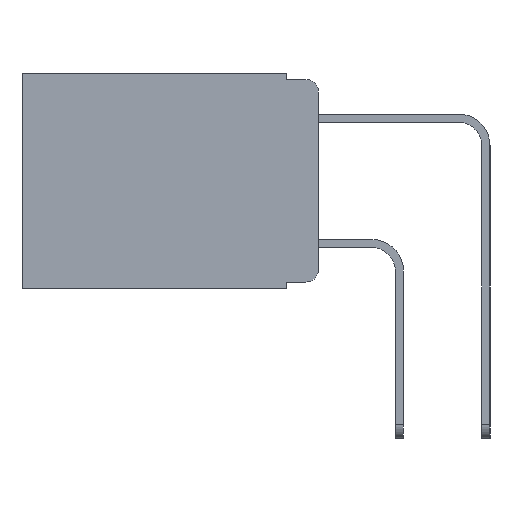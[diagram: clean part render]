
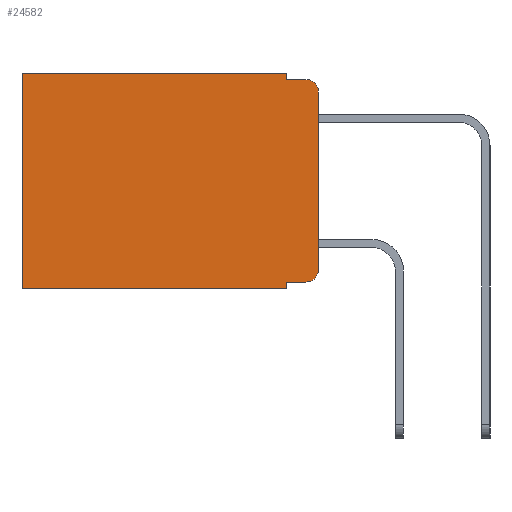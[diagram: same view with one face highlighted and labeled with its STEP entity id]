
A CAD part, left-side view. The second image highlights one B-rep face of the part: STEP entity #24582.
In plain terms, the highlighted planar face has unit normal (-1, 0, 0).
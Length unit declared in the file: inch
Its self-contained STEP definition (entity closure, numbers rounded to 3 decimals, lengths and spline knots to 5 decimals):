
#254 = PLANE ( 'NONE',  #23948 ) ;
#559 = LINE ( 'NONE', #24559, #5121 ) ;
#582 = VECTOR ( 'NONE', #24041, 39.37008 ) ;
#994 = EDGE_CURVE ( 'NONE', #19160, #9519, #16504, .T. ) ;
#1526 = DIRECTION ( 'NONE',  ( 0., 0., -1. ) ) ;
#1638 = EDGE_LOOP ( 'NONE', ( #12929, #13010, #13178, #13196, #13227, #13409, #13428, #13522, #13635, #13654 ) ) ;
#1689 = FACE_OUTER_BOUND ( 'NONE', #1638, .T. ) ;
#1794 = DIRECTION ( 'NONE',  ( -1., 0., 0. ) ) ;
#2107 = VERTEX_POINT ( 'NONE', #8570 ) ;
#2148 = CARTESIAN_POINT ( 'NONE',  ( 0.298, 0.051, 0. ) ) ;
#2186 = AXIS2_PLACEMENT_3D ( 'NONE', #14984, #3344, #16945 ) ;
#2248 = DIRECTION ( 'NONE',  ( 1., 0., 0. ) ) ;
#2664 = VECTOR ( 'NONE', #23885, 39.37008 ) ;
#2675 = CARTESIAN_POINT ( 'NONE',  ( 0.298, 0.051, -0.333 ) ) ;
#2977 = EDGE_CURVE ( 'NONE', #10206, #17393, #21224, .T. ) ;
#2984 = CARTESIAN_POINT ( 'NONE',  ( 0.298, 0.051, -0.343 ) ) ;
#3323 = VECTOR ( 'NONE', #3538, 39.37008 ) ;
#3344 = DIRECTION ( 'NONE',  ( -1., 0., 0. ) ) ;
#3425 = EDGE_CURVE ( 'NONE', #9216, #24380, #559, .T. ) ;
#3452 = CARTESIAN_POINT ( 'NONE',  ( 0.298, 0.473, 0. ) ) ;
#3538 = DIRECTION ( 'NONE',  ( 0., 0., -1. ) ) ;
#3616 = EDGE_CURVE ( 'NONE', #2107, #9216, #21827, .T. ) ;
#4163 = EDGE_CURVE ( 'NONE', #9519, #13200, #4528, .T. ) ;
#4528 = LINE ( 'NONE', #11859, #19377 ) ;
#5121 = VECTOR ( 'NONE', #23825, 39.37008 ) ;
#6774 = VECTOR ( 'NONE', #1526, 39.37008 ) ;
#6919 = VECTOR ( 'NONE', #9480, 39.37008 ) ;
#7004 = VERTEX_POINT ( 'NONE', #14033 ) ;
#7548 = DIRECTION ( 'NONE',  ( 0., 0., -1. ) ) ;
#7786 = EDGE_CURVE ( 'NONE', #10090, #24380, #18799, .T. ) ;
#8004 = CARTESIAN_POINT ( 'NONE',  ( 0.298, 0., 0. ) ) ;
#8570 = CARTESIAN_POINT ( 'NONE',  ( 0.298, 0.051, -0.333 ) ) ;
#8912 = DIRECTION ( 'NONE',  ( 0., -1., 0. ) ) ;
#9122 = EDGE_CURVE ( 'NONE', #2107, #7004, #12995, .T. ) ;
#9209 = AXIS2_PLACEMENT_3D ( 'NONE', #13446, #1794, #15377 ) ;
#9216 = VERTEX_POINT ( 'NONE', #2984 ) ;
#9480 = DIRECTION ( 'NONE',  ( 0., 1., 0. ) ) ;
#9519 = VERTEX_POINT ( 'NONE', #17422 ) ;
#10090 = VERTEX_POINT ( 'NONE', #3452 ) ;
#10206 = VERTEX_POINT ( 'NONE', #23145 ) ;
#11327 = CARTESIAN_POINT ( 'NONE',  ( 0.298, 0.051, 0. ) ) ;
#11859 = CARTESIAN_POINT ( 'NONE',  ( 0.298, 0.051, -0.01 ) ) ;
#11929 = EDGE_CURVE ( 'NONE', #10206, #13200, #16487, .T. ) ;
#12929 = ORIENTED_EDGE ( 'NONE', *, *, #2977, .F. ) ;
#12995 = LINE ( 'NONE', #2675, #2664 ) ;
#13010 = ORIENTED_EDGE ( 'NONE', *, *, #11929, .T. ) ;
#13178 = ORIENTED_EDGE ( 'NONE', *, *, #4163, .F. ) ;
#13196 = ORIENTED_EDGE ( 'NONE', *, *, #994, .F. ) ;
#13200 = VERTEX_POINT ( 'NONE', #17282 ) ;
#13217 = CARTESIAN_POINT ( 'NONE',  ( 0.298, 0.473, -0.343 ) ) ;
#13227 = ORIENTED_EDGE ( 'NONE', *, *, #23196, .T. ) ;
#13409 = ORIENTED_EDGE ( 'NONE', *, *, #7786, .T. ) ;
#13428 = ORIENTED_EDGE ( 'NONE', *, *, #3425, .F. ) ;
#13446 = CARTESIAN_POINT ( 'NONE',  ( 0.298, 0.02, -0.03 ) ) ;
#13522 = ORIENTED_EDGE ( 'NONE', *, *, #3616, .F. ) ;
#13635 = ORIENTED_EDGE ( 'NONE', *, *, #9122, .T. ) ;
#13654 = ORIENTED_EDGE ( 'NONE', *, *, #19983, .T. ) ;
#14033 = CARTESIAN_POINT ( 'NONE',  ( 0.298, 0.02, -0.333 ) ) ;
#14984 = CARTESIAN_POINT ( 'NONE',  ( 0.298, 0.02, -0.313 ) ) ;
#15377 = DIRECTION ( 'NONE',  ( 0., 0., -1. ) ) ;
#15808 = DIRECTION ( 'NONE',  ( 0., 0., -1. ) ) ;
#16487 = CIRCLE ( 'NONE', #9209, 0.02 ) ;
#16504 = LINE ( 'NONE', #11327, #6774 ) ;
#16719 = VECTOR ( 'NONE', #7548, 39.37008 ) ;
#16945 = DIRECTION ( 'NONE',  ( 0., 0., -1. ) ) ;
#17272 = LINE ( 'NONE', #22963, #6919 ) ;
#17282 = CARTESIAN_POINT ( 'NONE',  ( 0.298, 0.02, -0.01 ) ) ;
#17393 = VERTEX_POINT ( 'NONE', #17919 ) ;
#17422 = CARTESIAN_POINT ( 'NONE',  ( 0.298, 0.051, -0.01 ) ) ;
#17919 = CARTESIAN_POINT ( 'NONE',  ( 0.298, 0., -0.313 ) ) ;
#18799 = LINE ( 'NONE', #20908, #3323 ) ;
#19160 = VERTEX_POINT ( 'NONE', #2148 ) ;
#19377 = VECTOR ( 'NONE', #8912, 39.37008 ) ;
#19983 = EDGE_CURVE ( 'NONE', #7004, #17393, #23720, .T. ) ;
#20908 = CARTESIAN_POINT ( 'NONE',  ( 0.298, 0.473, 0. ) ) ;
#21224 = LINE ( 'NONE', #24872, #582 ) ;
#21820 = CARTESIAN_POINT ( 'NONE',  ( 0.298, 0.051, 0. ) ) ;
#21827 = LINE ( 'NONE', #21820, #16719 ) ;
#22963 = CARTESIAN_POINT ( 'NONE',  ( 0.298, 0., 0. ) ) ;
#23145 = CARTESIAN_POINT ( 'NONE',  ( 0.298, 0., -0.03 ) ) ;
#23196 = EDGE_CURVE ( 'NONE', #19160, #10090, #17272, .T. ) ;
#23720 = CIRCLE ( 'NONE', #2186, 0.02 ) ;
#23825 = DIRECTION ( 'NONE',  ( 0., 1., 0. ) ) ;
#23885 = DIRECTION ( 'NONE',  ( 0., -1., 0. ) ) ;
#23948 = AXIS2_PLACEMENT_3D ( 'NONE', #8004, #2248, #15808 ) ;
#24041 = DIRECTION ( 'NONE',  ( 0., 0., -1. ) ) ;
#24380 = VERTEX_POINT ( 'NONE', #13217 ) ;
#24559 = CARTESIAN_POINT ( 'NONE',  ( 0.298, 0., -0.343 ) ) ;
#24582 = ADVANCED_FACE ( 'NONE', ( #1689 ), #254, .F. ) ;
#24872 = CARTESIAN_POINT ( 'NONE',  ( 0.298, 0., 0. ) ) ;
